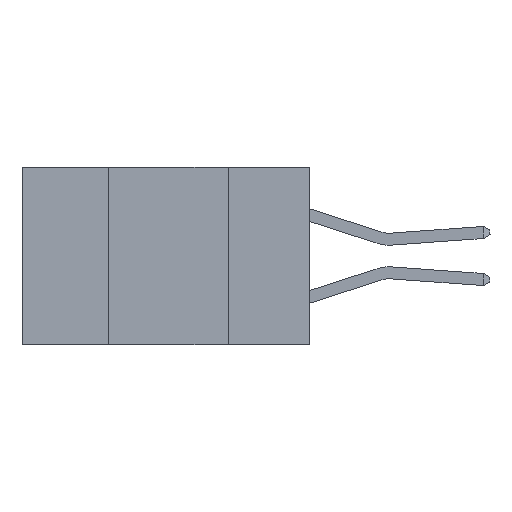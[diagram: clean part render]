
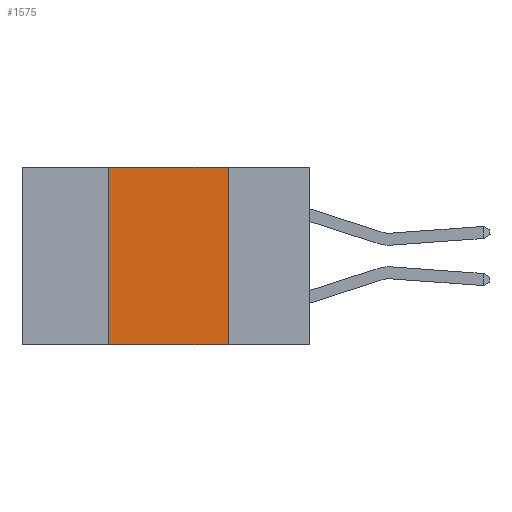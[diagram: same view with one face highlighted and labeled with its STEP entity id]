
A CAD part, left-side view. The second image highlights one B-rep face of the part: STEP entity #1575.
In plain terms, the highlighted planar face has unit normal (-1, 0, 0).
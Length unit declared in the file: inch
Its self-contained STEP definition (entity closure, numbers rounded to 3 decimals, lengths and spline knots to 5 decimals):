
#138 = EDGE_CURVE ( 'NONE', #7846, #5507, #5102, .T. ) ;
#305 = PLANE ( 'NONE',  #8863 ) ;
#463 = DIRECTION ( 'NONE',  ( 0., 0., -1. ) ) ;
#604 = DIRECTION ( 'NONE',  ( 0., 0., 1. ) ) ;
#984 = DIRECTION ( 'NONE',  ( 0., -1., 0. ) ) ;
#1149 = DIRECTION ( 'NONE',  ( 1., 0., 0. ) ) ;
#1575 = ADVANCED_FACE ( 'NONE', ( #4465 ), #305, .F. ) ;
#1660 = ORIENTED_EDGE ( 'NONE', *, *, #7910, .F. ) ;
#1840 = VERTEX_POINT ( 'NONE', #9966 ) ;
#2160 = VECTOR ( 'NONE', #3306, 39.37008 ) ;
#2371 = EDGE_LOOP ( 'NONE', ( #1660, #8181, #9295, #4809 ) ) ;
#3306 = DIRECTION ( 'NONE',  ( 0., 0., -1. ) ) ;
#3584 = VECTOR ( 'NONE', #4471, 39.37008 ) ;
#4465 = FACE_OUTER_BOUND ( 'NONE', #2371, .T. ) ;
#4471 = DIRECTION ( 'NONE',  ( 0., -1., 0. ) ) ;
#4809 = ORIENTED_EDGE ( 'NONE', *, *, #138, .T. ) ;
#5102 = LINE ( 'NONE', #9484, #3584 ) ;
#5123 = LINE ( 'NONE', #6849, #8651 ) ;
#5507 = VERTEX_POINT ( 'NONE', #7146 ) ;
#6060 = VERTEX_POINT ( 'NONE', #9947 ) ;
#6362 = CARTESIAN_POINT ( 'NONE',  ( 0., 0.42, -0.37 ) ) ;
#6834 = EDGE_CURVE ( 'NONE', #7846, #6060, #9035, .T. ) ;
#6849 = CARTESIAN_POINT ( 'NONE',  ( 0., 0.6, 0. ) ) ;
#6873 = VECTOR ( 'NONE', #604, 39.37008 ) ;
#6971 = CARTESIAN_POINT ( 'NONE',  ( 0., 0.6, 0. ) ) ;
#7146 = CARTESIAN_POINT ( 'NONE',  ( 0., 0.17, -0.37 ) ) ;
#7373 = LINE ( 'NONE', #7533, #2160 ) ;
#7533 = CARTESIAN_POINT ( 'NONE',  ( 0., 0.17, -0.37 ) ) ;
#7846 = VERTEX_POINT ( 'NONE', #10485 ) ;
#7910 = EDGE_CURVE ( 'NONE', #1840, #5507, #7373, .T. ) ;
#8181 = ORIENTED_EDGE ( 'NONE', *, *, #9184, .F. ) ;
#8651 = VECTOR ( 'NONE', #984, 39.37008 ) ;
#8863 = AXIS2_PLACEMENT_3D ( 'NONE', #6971, #1149, #463 ) ;
#9035 = LINE ( 'NONE', #6362, #6873 ) ;
#9184 = EDGE_CURVE ( 'NONE', #6060, #1840, #5123, .T. ) ;
#9295 = ORIENTED_EDGE ( 'NONE', *, *, #6834, .F. ) ;
#9484 = CARTESIAN_POINT ( 'NONE',  ( 0., 0.6, -0.37 ) ) ;
#9947 = CARTESIAN_POINT ( 'NONE',  ( 0., 0.42, 0. ) ) ;
#9966 = CARTESIAN_POINT ( 'NONE',  ( 0., 0.17, 0. ) ) ;
#10485 = CARTESIAN_POINT ( 'NONE',  ( 0., 0.42, -0.37 ) ) ;
